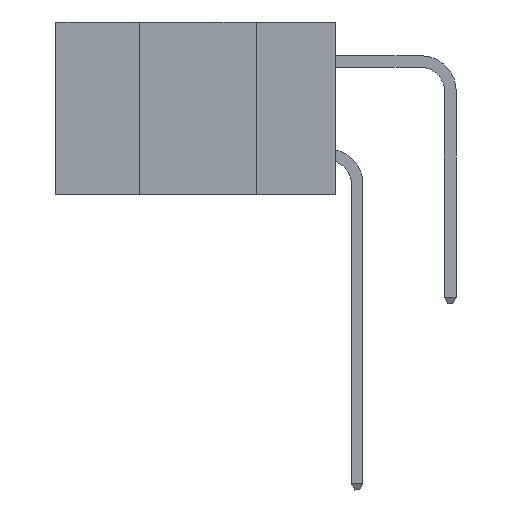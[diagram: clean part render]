
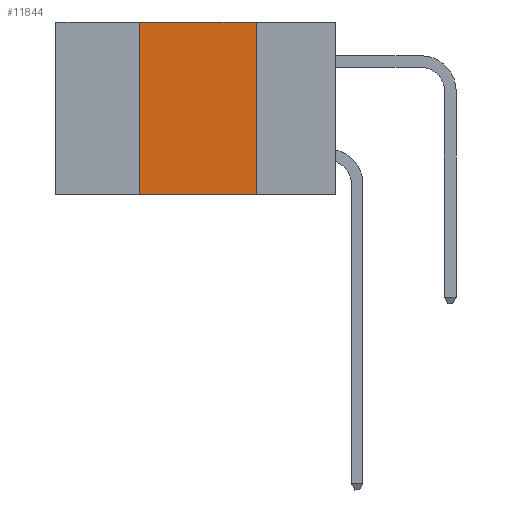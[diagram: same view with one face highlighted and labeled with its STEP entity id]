
A CAD part, left-side view. The second image highlights one B-rep face of the part: STEP entity #11844.
In plain terms, the highlighted planar face has unit normal (-1, 0, 0).
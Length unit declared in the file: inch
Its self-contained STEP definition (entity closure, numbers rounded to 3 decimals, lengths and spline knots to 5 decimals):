
#88 = CARTESIAN_POINT ( 'NONE',  ( 0., 0.42, 0. ) ) ;
#780 = EDGE_CURVE ( 'NONE', #30046, #16109, #4938, .T. ) ;
#1126 = VECTOR ( 'NONE', #12915, 39.37008 ) ;
#2421 = EDGE_LOOP ( 'NONE', ( #18022, #7139, #33948, #35267 ) ) ;
#4777 = LINE ( 'NONE', #18332, #18348 ) ;
#4938 = LINE ( 'NONE', #31832, #1126 ) ;
#5738 = CARTESIAN_POINT ( 'NONE',  ( 0., 0.17, -0.37 ) ) ;
#7139 = ORIENTED_EDGE ( 'NONE', *, *, #28985, .F. ) ;
#7647 = FACE_OUTER_BOUND ( 'NONE', #2421, .T. ) ;
#7687 = CARTESIAN_POINT ( 'NONE',  ( 0., 0.6, -0.37 ) ) ;
#7689 = VERTEX_POINT ( 'NONE', #5738 ) ;
#8788 = CARTESIAN_POINT ( 'NONE',  ( 0., 0.6, 0. ) ) ;
#11176 = DIRECTION ( 'NONE',  ( 0., -1., 0. ) ) ;
#11844 = ADVANCED_FACE ( 'NONE', ( #7647 ), #27007, .F. ) ;
#12915 = DIRECTION ( 'NONE',  ( 0., 0., 1. ) ) ;
#14973 = DIRECTION ( 'NONE',  ( 1., 0., 0. ) ) ;
#16109 = VERTEX_POINT ( 'NONE', #88 ) ;
#16318 = DIRECTION ( 'NONE',  ( 0., 0., -1. ) ) ;
#18022 = ORIENTED_EDGE ( 'NONE', *, *, #27568, .F. ) ;
#18332 = CARTESIAN_POINT ( 'NONE',  ( 0., 0.6, 0. ) ) ;
#18348 = VECTOR ( 'NONE', #24550, 39.37008 ) ;
#18749 = CARTESIAN_POINT ( 'NONE',  ( 0., 0.17, 0. ) ) ;
#20069 = AXIS2_PLACEMENT_3D ( 'NONE', #8788, #14973, #36613 ) ;
#23629 = CARTESIAN_POINT ( 'NONE',  ( 0., 0.42, -0.37 ) ) ;
#24550 = DIRECTION ( 'NONE',  ( 0., -1., 0. ) ) ;
#25642 = EDGE_CURVE ( 'NONE', #30046, #7689, #31645, .T. ) ;
#25774 = CARTESIAN_POINT ( 'NONE',  ( 0., 0.17, 0. ) ) ;
#26340 = VECTOR ( 'NONE', #11176, 39.37008 ) ;
#27007 = PLANE ( 'NONE',  #20069 ) ;
#27568 = EDGE_CURVE ( 'NONE', #39542, #7689, #31959, .T. ) ;
#28590 = VECTOR ( 'NONE', #16318, 39.37008 ) ;
#28985 = EDGE_CURVE ( 'NONE', #16109, #39542, #4777, .T. ) ;
#30046 = VERTEX_POINT ( 'NONE', #23629 ) ;
#31645 = LINE ( 'NONE', #7687, #26340 ) ;
#31832 = CARTESIAN_POINT ( 'NONE',  ( 0., 0.42, 0. ) ) ;
#31959 = LINE ( 'NONE', #25774, #28590 ) ;
#33948 = ORIENTED_EDGE ( 'NONE', *, *, #780, .F. ) ;
#35267 = ORIENTED_EDGE ( 'NONE', *, *, #25642, .T. ) ;
#36613 = DIRECTION ( 'NONE',  ( 0., 0., -1. ) ) ;
#39542 = VERTEX_POINT ( 'NONE', #18749 ) ;
